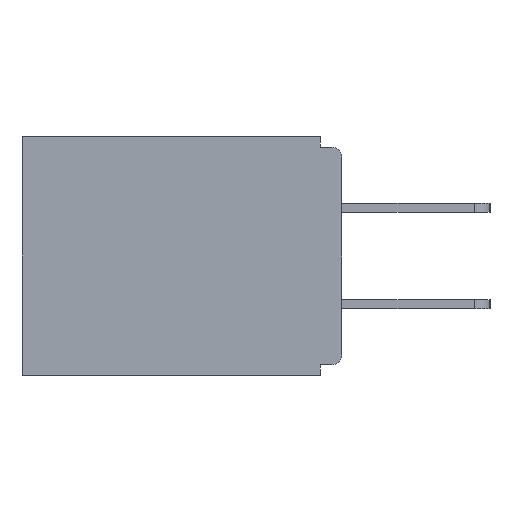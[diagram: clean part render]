
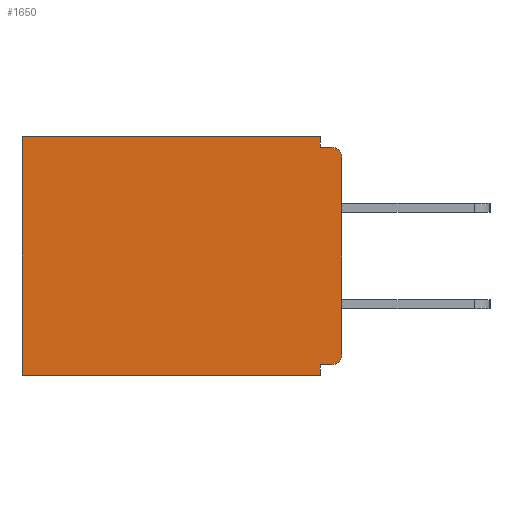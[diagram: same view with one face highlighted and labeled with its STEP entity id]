
A CAD part, left-side view. The second image highlights one B-rep face of the part: STEP entity #1650.
In plain terms, the highlighted planar face has unit normal (-1, 0, 0).
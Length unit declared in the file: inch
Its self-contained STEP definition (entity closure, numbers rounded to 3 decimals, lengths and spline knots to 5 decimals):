
#28 = EDGE_CURVE ( 'NONE', #4832, #8071, #4512, .T. ) ;
#139 = DIRECTION ( 'NONE',  ( 0., 0., -1. ) ) ;
#158 = VECTOR ( 'NONE', #9326, 39.37008 ) ;
#576 = CARTESIAN_POINT ( 'NONE',  ( 0.298, 0.46, -0.343 ) ) ;
#604 = CARTESIAN_POINT ( 'NONE',  ( 0.298, 0.015, -0.015 ) ) ;
#634 = VERTEX_POINT ( 'NONE', #604 ) ;
#740 = ORIENTED_EDGE ( 'NONE', *, *, #951, .F. ) ;
#768 = VERTEX_POINT ( 'NONE', #2450 ) ;
#824 = ORIENTED_EDGE ( 'NONE', *, *, #7628, .T. ) ;
#909 = CARTESIAN_POINT ( 'NONE',  ( 0.298, 0.031, 0. ) ) ;
#951 = EDGE_CURVE ( 'NONE', #5628, #768, #10304, .T. ) ;
#1020 = DIRECTION ( 'NONE',  ( -1., 0., 0. ) ) ;
#1189 = EDGE_CURVE ( 'NONE', #3295, #5628, #9062, .T. ) ;
#1305 = ORIENTED_EDGE ( 'NONE', *, *, #6605, .T. ) ;
#1352 = DIRECTION ( 'NONE',  ( 0., 0., -1. ) ) ;
#1397 = LINE ( 'NONE', #6686, #158 ) ;
#1408 = DIRECTION ( 'NONE',  ( 0., 1., 0. ) ) ;
#1650 = ADVANCED_FACE ( 'NONE', ( #6578 ), #5802, .F. ) ;
#2003 = VECTOR ( 'NONE', #7161, 39.37008 ) ;
#2028 = VERTEX_POINT ( 'NONE', #3938 ) ;
#2296 = VECTOR ( 'NONE', #3704, 39.37008 ) ;
#2450 = CARTESIAN_POINT ( 'NONE',  ( 0.298, 0.031, -0.343 ) ) ;
#2583 = CARTESIAN_POINT ( 'NONE',  ( 0.298, 0., -0.313 ) ) ;
#2645 = CARTESIAN_POINT ( 'NONE',  ( 0.298, 0., -0.03 ) ) ;
#2757 = LINE ( 'NONE', #6582, #7901 ) ;
#3295 = VERTEX_POINT ( 'NONE', #11084 ) ;
#3417 = LINE ( 'NONE', #6366, #2296 ) ;
#3704 = DIRECTION ( 'NONE',  ( 0., 0., -1. ) ) ;
#3938 = CARTESIAN_POINT ( 'NONE',  ( 0.298, 0.031, -0.015 ) ) ;
#3989 = LINE ( 'NONE', #5932, #8828 ) ;
#4055 = CARTESIAN_POINT ( 'NONE',  ( 0.298, 0., 0. ) ) ;
#4512 = LINE ( 'NONE', #8894, #2003 ) ;
#4521 = DIRECTION ( 'NONE',  ( 0., 0., -1. ) ) ;
#4597 = EDGE_CURVE ( 'NONE', #2028, #634, #1397, .T. ) ;
#4790 = EDGE_LOOP ( 'NONE', ( #1305, #8800, #4921, #10819, #10353, #5653, #740, #9974, #824, #5501 ) ) ;
#4832 = VERTEX_POINT ( 'NONE', #2645 ) ;
#4921 = ORIENTED_EDGE ( 'NONE', *, *, #6447, .F. ) ;
#5501 = ORIENTED_EDGE ( 'NONE', *, *, #28, .F. ) ;
#5580 = CARTESIAN_POINT ( 'NONE',  ( 0.298, 0.031, -0.328 ) ) ;
#5628 = VERTEX_POINT ( 'NONE', #5580 ) ;
#5653 = ORIENTED_EDGE ( 'NONE', *, *, #10646, .F. ) ;
#5802 = PLANE ( 'NONE',  #9490 ) ;
#5932 = CARTESIAN_POINT ( 'NONE',  ( 0.298, 0.031, -0.343 ) ) ;
#6154 = DIRECTION ( 'NONE',  ( 0., 1., 0. ) ) ;
#6254 = DIRECTION ( 'NONE',  ( -1., 0., 0. ) ) ;
#6328 = CARTESIAN_POINT ( 'NONE',  ( 0.298, 0.015, -0.313 ) ) ;
#6342 = EDGE_CURVE ( 'NONE', #8921, #9214, #3417, .T. ) ;
#6366 = CARTESIAN_POINT ( 'NONE',  ( 0.298, 0.46, 0. ) ) ;
#6447 = EDGE_CURVE ( 'NONE', #7607, #2028, #3989, .T. ) ;
#6578 = FACE_OUTER_BOUND ( 'NONE', #4790, .T. ) ;
#6582 = CARTESIAN_POINT ( 'NONE',  ( 0.298, 0., -0.343 ) ) ;
#6597 = DIRECTION ( 'NONE',  ( 1., 0., 0. ) ) ;
#6605 = EDGE_CURVE ( 'NONE', #4832, #634, #10895, .T. ) ;
#6683 = CARTESIAN_POINT ( 'NONE',  ( 0.298, 0., -0.328 ) ) ;
#6686 = CARTESIAN_POINT ( 'NONE',  ( 0.298, 0., -0.015 ) ) ;
#7161 = DIRECTION ( 'NONE',  ( 0., 0., -1. ) ) ;
#7607 = VERTEX_POINT ( 'NONE', #909 ) ;
#7617 = CARTESIAN_POINT ( 'NONE',  ( 0.298, 0.46, 0. ) ) ;
#7628 = EDGE_CURVE ( 'NONE', #3295, #8071, #8803, .T. ) ;
#7901 = VECTOR ( 'NONE', #6154, 39.37008 ) ;
#8071 = VERTEX_POINT ( 'NONE', #2583 ) ;
#8096 = VECTOR ( 'NONE', #10326, 39.37008 ) ;
#8402 = EDGE_CURVE ( 'NONE', #7607, #8921, #9203, .T. ) ;
#8480 = AXIS2_PLACEMENT_3D ( 'NONE', #6328, #1020, #8857 ) ;
#8508 = CARTESIAN_POINT ( 'NONE',  ( 0.298, 0., 0. ) ) ;
#8778 = VECTOR ( 'NONE', #139, 39.37008 ) ;
#8800 = ORIENTED_EDGE ( 'NONE', *, *, #4597, .F. ) ;
#8803 = CIRCLE ( 'NONE', #8480, 0.015 ) ;
#8828 = VECTOR ( 'NONE', #9479, 39.37008 ) ;
#8857 = DIRECTION ( 'NONE',  ( 0., 0., -1. ) ) ;
#8894 = CARTESIAN_POINT ( 'NONE',  ( 0.298, 0., 0. ) ) ;
#8897 = CARTESIAN_POINT ( 'NONE',  ( 0.298, 0.015, -0.03 ) ) ;
#8921 = VERTEX_POINT ( 'NONE', #7617 ) ;
#8954 = CARTESIAN_POINT ( 'NONE',  ( 0.298, 0.031, -0.343 ) ) ;
#9062 = LINE ( 'NONE', #6683, #9893 ) ;
#9203 = LINE ( 'NONE', #8508, #8096 ) ;
#9214 = VERTEX_POINT ( 'NONE', #576 ) ;
#9326 = DIRECTION ( 'NONE',  ( 0., -1., 0. ) ) ;
#9479 = DIRECTION ( 'NONE',  ( 0., 0., -1. ) ) ;
#9490 = AXIS2_PLACEMENT_3D ( 'NONE', #4055, #6597, #1352 ) ;
#9684 = AXIS2_PLACEMENT_3D ( 'NONE', #8897, #6254, #4521 ) ;
#9893 = VECTOR ( 'NONE', #1408, 39.37008 ) ;
#9974 = ORIENTED_EDGE ( 'NONE', *, *, #1189, .F. ) ;
#10304 = LINE ( 'NONE', #8954, #8778 ) ;
#10326 = DIRECTION ( 'NONE',  ( 0., 1., 0. ) ) ;
#10353 = ORIENTED_EDGE ( 'NONE', *, *, #6342, .T. ) ;
#10646 = EDGE_CURVE ( 'NONE', #768, #9214, #2757, .T. ) ;
#10819 = ORIENTED_EDGE ( 'NONE', *, *, #8402, .T. ) ;
#10895 = CIRCLE ( 'NONE', #9684, 0.015 ) ;
#11084 = CARTESIAN_POINT ( 'NONE',  ( 0.298, 0.015, -0.328 ) ) ;
